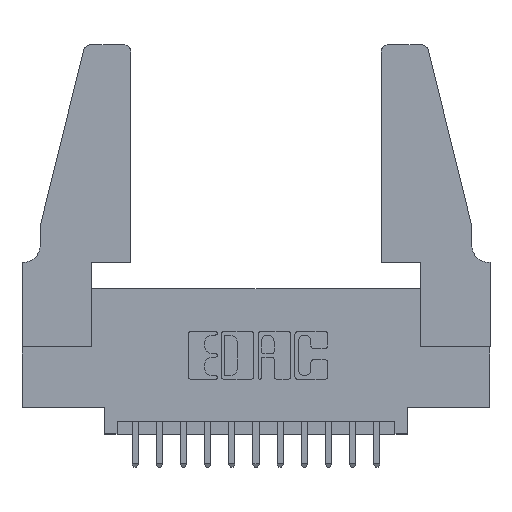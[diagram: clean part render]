
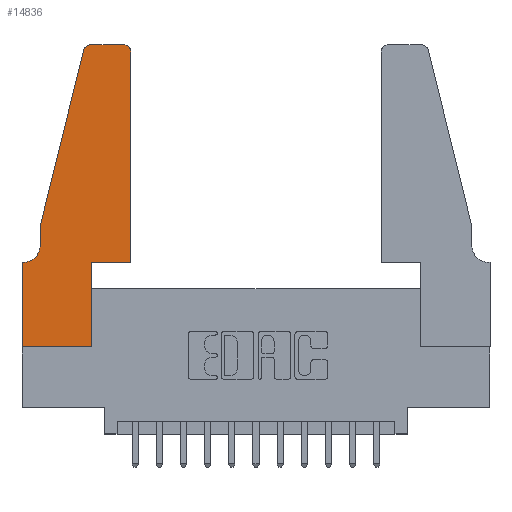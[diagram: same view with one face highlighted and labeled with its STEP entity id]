
A CAD part, top view. The second image highlights one B-rep face of the part: STEP entity #14836.
In plain terms, the highlighted planar face has unit normal (0, 0, 1).
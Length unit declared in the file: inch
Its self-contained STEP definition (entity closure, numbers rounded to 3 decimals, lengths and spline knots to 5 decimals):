
#76 = AXIS2_PLACEMENT_3D ( 'NONE', #8555, #1766, #497 ) ;
#231 = VECTOR ( 'NONE', #14684, 39.37008 ) ;
#271 = EDGE_CURVE ( 'NONE', #5778, #13188, #9336, .T. ) ;
#497 = DIRECTION ( 'NONE',  ( 1., 0., 0. ) ) ;
#546 = ORIENTED_EDGE ( 'NONE', *, *, #13087, .T. ) ;
#871 = LINE ( 'NONE', #930, #12019 ) ;
#923 = CARTESIAN_POINT ( 'NONE',  ( 0., 0.35, 0.37 ) ) ;
#930 = CARTESIAN_POINT ( 'NONE',  ( 0.4505, 0.35, 0.37 ) ) ;
#1070 = DIRECTION ( 'NONE',  ( 1., 0., 0. ) ) ;
#1766 = DIRECTION ( 'NONE',  ( 0., 0., 1. ) ) ;
#1898 = ORIENTED_EDGE ( 'NONE', *, *, #271, .T. ) ;
#2015 = EDGE_CURVE ( 'NONE', #9182, #5778, #7066, .T. ) ;
#2095 = VERTEX_POINT ( 'NONE', #12198 ) ;
#2429 = DIRECTION ( 'NONE',  ( 0., -1., 0. ) ) ;
#3166 = LINE ( 'NONE', #5220, #5555 ) ;
#3228 = VERTEX_POINT ( 'NONE', #11510 ) ;
#3285 = DIRECTION ( 'NONE',  ( 1., 0., 0. ) ) ;
#3349 = VECTOR ( 'NONE', #12868, 39.37008 ) ;
#3375 = CARTESIAN_POINT ( 'NONE',  ( 0.4505, 1.22, 0.37 ) ) ;
#3379 = DIRECTION ( 'NONE',  ( 0., 0., 1. ) ) ;
#3517 = VECTOR ( 'NONE', #6988, 39.37008 ) ;
#3518 = EDGE_CURVE ( 'NONE', #7720, #2095, #11077, .T. ) ;
#3584 = CARTESIAN_POINT ( 'NONE',  ( 0.284, 1.25, 0.37 ) ) ;
#3815 = DIRECTION ( 'NONE',  ( 0., -1., 0. ) ) ;
#3867 = CARTESIAN_POINT ( 'NONE',  ( 0.0755, 0.35, 0.37 ) ) ;
#4042 = AXIS2_PLACEMENT_3D ( 'NONE', #6448, #13476, #4082 ) ;
#4082 = DIRECTION ( 'NONE',  ( -1., 0., 0. ) ) ;
#4117 = EDGE_CURVE ( 'NONE', #13188, #5478, #10334, .T. ) ;
#4165 = CARTESIAN_POINT ( 'NONE',  ( 0.2865, 0.35, 0.37 ) ) ;
#4319 = VECTOR ( 'NONE', #3815, 39.37008 ) ;
#4363 = DIRECTION ( 'NONE',  ( -1., 0., 0. ) ) ;
#4465 = FACE_OUTER_BOUND ( 'NONE', #10065, .T. ) ;
#4608 = DIRECTION ( 'NONE',  ( 1., 0., 0. ) ) ;
#4881 = EDGE_CURVE ( 'NONE', #11740, #5064, #9028, .T. ) ;
#4900 = ORIENTED_EDGE ( 'NONE', *, *, #10584, .T. ) ;
#5064 = VERTEX_POINT ( 'NONE', #6966 ) ;
#5220 = CARTESIAN_POINT ( 'NONE',  ( 0.0755, 0.5, 0.37 ) ) ;
#5339 = ORIENTED_EDGE ( 'NONE', *, *, #3518, .T. ) ;
#5478 = VERTEX_POINT ( 'NONE', #14918 ) ;
#5497 = CARTESIAN_POINT ( 'NONE',  ( 0.0755, 0.5, 0.37 ) ) ;
#5555 = VECTOR ( 'NONE', #12619, 39.37008 ) ;
#5778 = VERTEX_POINT ( 'NONE', #11407 ) ;
#5936 = CARTESIAN_POINT ( 'NONE',  ( 0., 0., 0.37 ) ) ;
#5940 = EDGE_CURVE ( 'NONE', #10302, #12798, #6421, .T. ) ;
#6172 = ORIENTED_EDGE ( 'NONE', *, *, #11002, .T. ) ;
#6421 = CIRCLE ( 'NONE', #6845, 0.03 ) ;
#6448 = CARTESIAN_POINT ( 'NONE',  ( 0.0055, 0.42, 0.37 ) ) ;
#6465 = LINE ( 'NONE', #9345, #3349 ) ;
#6678 = LINE ( 'NONE', #13386, #10879 ) ;
#6820 = CARTESIAN_POINT ( 'NONE',  ( 0., 0.35, 0.37 ) ) ;
#6845 = AXIS2_PLACEMENT_3D ( 'NONE', #8157, #11561, #1070 ) ;
#6887 = ORIENTED_EDGE ( 'NONE', *, *, #5940, .T. ) ;
#6966 = CARTESIAN_POINT ( 'NONE',  ( 0.4205, 1.25, 0.37 ) ) ;
#6988 = DIRECTION ( 'NONE',  ( -1., 0., 0. ) ) ;
#7066 = LINE ( 'NONE', #5936, #10746 ) ;
#7407 = CARTESIAN_POINT ( 'NONE',  ( 0.0755, 0.5, 0.37 ) ) ;
#7720 = VERTEX_POINT ( 'NONE', #5497 ) ;
#8033 = CARTESIAN_POINT ( 'NONE',  ( 0., 0., 0.37 ) ) ;
#8157 = CARTESIAN_POINT ( 'NONE',  ( 0.284, 1.22, 0.37 ) ) ;
#8331 = EDGE_CURVE ( 'NONE', #5478, #11450, #871, .T. ) ;
#8555 = CARTESIAN_POINT ( 'NONE',  ( 0.4205, 1.22, 0.37 ) ) ;
#8636 = ORIENTED_EDGE ( 'NONE', *, *, #4881, .T. ) ;
#9028 = CIRCLE ( 'NONE', #76, 0.03 ) ;
#9182 = VERTEX_POINT ( 'NONE', #923 ) ;
#9336 = LINE ( 'NONE', #8033, #10605 ) ;
#9345 = CARTESIAN_POINT ( 'NONE',  ( 0.4505, 0.35, 0.37 ) ) ;
#9974 = ORIENTED_EDGE ( 'NONE', *, *, #10604, .T. ) ;
#10065 = EDGE_LOOP ( 'NONE', ( #12293, #6887, #4900, #5339, #546, #6172, #12793, #1898, #11249, #10559, #9974, #8636 ) ) ;
#10147 = EDGE_CURVE ( 'NONE', #5064, #10302, #6678, .T. ) ;
#10290 = PLANE ( 'NONE',  #12508 ) ;
#10302 = VERTEX_POINT ( 'NONE', #3584 ) ;
#10334 = LINE ( 'NONE', #4165, #231 ) ;
#10482 = DIRECTION ( 'NONE',  ( 1., 0., 0. ) ) ;
#10559 = ORIENTED_EDGE ( 'NONE', *, *, #8331, .T. ) ;
#10584 = EDGE_CURVE ( 'NONE', #12798, #7720, #3166, .T. ) ;
#10604 = EDGE_CURVE ( 'NONE', #11450, #11740, #6465, .T. ) ;
#10605 = VECTOR ( 'NONE', #3285, 39.37008 ) ;
#10746 = VECTOR ( 'NONE', #2429, 39.37008 ) ;
#10879 = VECTOR ( 'NONE', #4363, 39.37008 ) ;
#11002 = EDGE_CURVE ( 'NONE', #3228, #9182, #15034, .T. ) ;
#11077 = LINE ( 'NONE', #7407, #4319 ) ;
#11249 = ORIENTED_EDGE ( 'NONE', *, *, #4117, .T. ) ;
#11407 = CARTESIAN_POINT ( 'NONE',  ( 0., 0., 0.37 ) ) ;
#11450 = VERTEX_POINT ( 'NONE', #12506 ) ;
#11510 = CARTESIAN_POINT ( 'NONE',  ( 0.0055, 0.35, 0.37 ) ) ;
#11561 = DIRECTION ( 'NONE',  ( 0., 0., 1. ) ) ;
#11713 = CARTESIAN_POINT ( 'NONE',  ( 0.2865, 0., 0.37 ) ) ;
#11740 = VERTEX_POINT ( 'NONE', #3375 ) ;
#12019 = VECTOR ( 'NONE', #10482, 39.37008 ) ;
#12198 = CARTESIAN_POINT ( 'NONE',  ( 0.0755, 0.42, 0.37 ) ) ;
#12293 = ORIENTED_EDGE ( 'NONE', *, *, #10147, .T. ) ;
#12506 = CARTESIAN_POINT ( 'NONE',  ( 0.4505, 0.35, 0.37 ) ) ;
#12508 = AXIS2_PLACEMENT_3D ( 'NONE', #6820, #3379, #4608 ) ;
#12619 = DIRECTION ( 'NONE',  ( -0.239, -0.971, 0. ) ) ;
#12793 = ORIENTED_EDGE ( 'NONE', *, *, #2015, .T. ) ;
#12798 = VERTEX_POINT ( 'NONE', #13379 ) ;
#12868 = DIRECTION ( 'NONE',  ( 0., 1., 0. ) ) ;
#13087 = EDGE_CURVE ( 'NONE', #2095, #3228, #13804, .T. ) ;
#13188 = VERTEX_POINT ( 'NONE', #11713 ) ;
#13379 = CARTESIAN_POINT ( 'NONE',  ( 0.25487, 1.22718, 0.37 ) ) ;
#13386 = CARTESIAN_POINT ( 'NONE',  ( 0.2605, 1.25, 0.37 ) ) ;
#13476 = DIRECTION ( 'NONE',  ( 0., 0., -1. ) ) ;
#13804 = CIRCLE ( 'NONE', #4042, 0.07 ) ;
#14684 = DIRECTION ( 'NONE',  ( 0., 1., 0. ) ) ;
#14836 = ADVANCED_FACE ( 'NONE', ( #4465 ), #10290, .T. ) ;
#14918 = CARTESIAN_POINT ( 'NONE',  ( 0.2865, 0.35, 0.37 ) ) ;
#15034 = LINE ( 'NONE', #3867, #3517 ) ;
